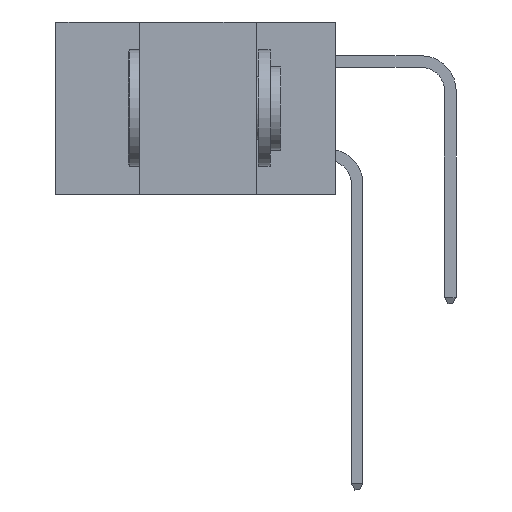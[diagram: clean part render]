
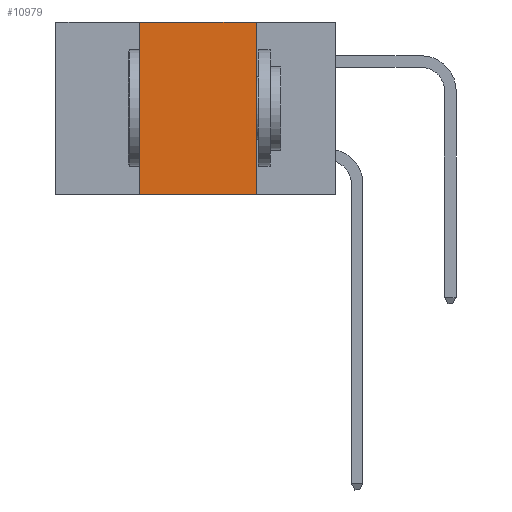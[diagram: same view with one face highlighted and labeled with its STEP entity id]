
A CAD part, left-side view. The second image highlights one B-rep face of the part: STEP entity #10979.
In plain terms, the highlighted planar face has unit normal (-1, 0, 0).
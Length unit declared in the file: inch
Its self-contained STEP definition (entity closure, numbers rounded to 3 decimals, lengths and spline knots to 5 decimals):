
#222 = CARTESIAN_POINT ( 'NONE',  ( 0., 0.6, 0. ) ) ;
#1177 = DIRECTION ( 'NONE',  ( 0., 0., -1. ) ) ;
#1199 = VECTOR ( 'NONE', #28663, 39.37008 ) ;
#2460 = CARTESIAN_POINT ( 'NONE',  ( 0., 0.17, -0.37 ) ) ;
#2985 = DIRECTION ( 'NONE',  ( 0., 0., -1. ) ) ;
#3988 = EDGE_CURVE ( 'NONE', #18143, #19964, #33381, .T. ) ;
#4892 = VERTEX_POINT ( 'NONE', #10900 ) ;
#5326 = VERTEX_POINT ( 'NONE', #2460 ) ;
#6285 = LINE ( 'NONE', #30083, #33372 ) ;
#7512 = CARTESIAN_POINT ( 'NONE',  ( 0., 0.42, 0. ) ) ;
#9103 = LINE ( 'NONE', #18170, #1199 ) ;
#9858 = FACE_OUTER_BOUND ( 'NONE', #18801, .T. ) ;
#10192 = EDGE_CURVE ( 'NONE', #18143, #5326, #9103, .T. ) ;
#10284 = ORIENTED_EDGE ( 'NONE', *, *, #30531, .F. ) ;
#10900 = CARTESIAN_POINT ( 'NONE',  ( 0., 0.17, 0. ) ) ;
#10979 = ADVANCED_FACE ( 'NONE', ( #9858 ), #16058, .F. ) ;
#11889 = ORIENTED_EDGE ( 'NONE', *, *, #3988, .F. ) ;
#12562 = DIRECTION ( 'NONE',  ( 0., -1., 0. ) ) ;
#12718 = ORIENTED_EDGE ( 'NONE', *, *, #10192, .T. ) ;
#15287 = DIRECTION ( 'NONE',  ( 0., 0., 1. ) ) ;
#16058 = PLANE ( 'NONE',  #25154 ) ;
#17698 = CARTESIAN_POINT ( 'NONE',  ( 0., 0.6, 0. ) ) ;
#18143 = VERTEX_POINT ( 'NONE', #26853 ) ;
#18170 = CARTESIAN_POINT ( 'NONE',  ( 0., 0.6, -0.37 ) ) ;
#18514 = EDGE_CURVE ( 'NONE', #19964, #4892, #31044, .T. ) ;
#18702 = DIRECTION ( 'NONE',  ( 1., 0., 0. ) ) ;
#18801 = EDGE_LOOP ( 'NONE', ( #10284, #32025, #11889, #12718 ) ) ;
#19964 = VERTEX_POINT ( 'NONE', #33067 ) ;
#24063 = VECTOR ( 'NONE', #12562, 39.37008 ) ;
#25154 = AXIS2_PLACEMENT_3D ( 'NONE', #222, #18702, #2985 ) ;
#25587 = VECTOR ( 'NONE', #15287, 39.37008 ) ;
#26853 = CARTESIAN_POINT ( 'NONE',  ( 0., 0.42, -0.37 ) ) ;
#28663 = DIRECTION ( 'NONE',  ( 0., -1., 0. ) ) ;
#30083 = CARTESIAN_POINT ( 'NONE',  ( 0., 0.17, 0. ) ) ;
#30531 = EDGE_CURVE ( 'NONE', #4892, #5326, #6285, .T. ) ;
#31044 = LINE ( 'NONE', #17698, #24063 ) ;
#32025 = ORIENTED_EDGE ( 'NONE', *, *, #18514, .F. ) ;
#33067 = CARTESIAN_POINT ( 'NONE',  ( 0., 0.42, 0. ) ) ;
#33372 = VECTOR ( 'NONE', #1177, 39.37008 ) ;
#33381 = LINE ( 'NONE', #7512, #25587 ) ;
